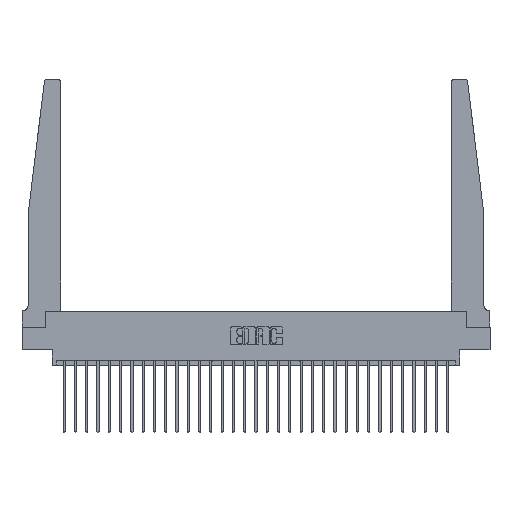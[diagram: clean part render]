
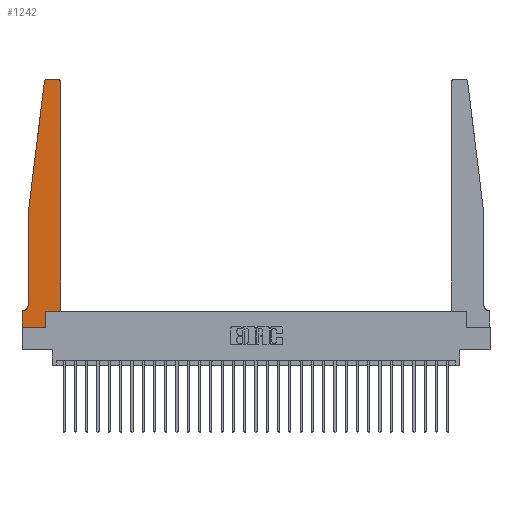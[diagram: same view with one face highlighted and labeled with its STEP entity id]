
A CAD part, top view. The second image highlights one B-rep face of the part: STEP entity #1242.
In plain terms, the highlighted planar face has unit normal (0, 0, 1).
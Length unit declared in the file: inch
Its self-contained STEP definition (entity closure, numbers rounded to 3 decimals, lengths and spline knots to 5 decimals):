
#350 = EDGE_CURVE ( 'NONE', #8178, #1044, #15282, .T. ) ;
#529 = VECTOR ( 'NONE', #13873, 39.37008 ) ;
#693 = LINE ( 'NONE', #27431, #7418 ) ;
#1044 = VERTEX_POINT ( 'NONE', #14270 ) ;
#1242 = ADVANCED_FACE ( 'NONE', ( #22518 ), #8789, .T. ) ;
#1253 = CARTESIAN_POINT ( 'NONE',  ( 0.065, 0.1875, 0.37 ) ) ;
#1385 = CARTESIAN_POINT ( 'NONE',  ( 0.425, 2.72, 0.37 ) ) ;
#1586 = AXIS2_PLACEMENT_3D ( 'NONE', #4360, #19884, #4650 ) ;
#1674 = AXIS2_PLACEMENT_3D ( 'NONE', #8197, #3888, #26198 ) ;
#1875 = CARTESIAN_POINT ( 'NONE',  ( 0.065, 1.25, 0.37 ) ) ;
#2654 = CARTESIAN_POINT ( 'NONE',  ( 0.24675, 2.72367, 0.37 ) ) ;
#2753 = CIRCLE ( 'NONE', #22094, 0.05 ) ;
#3309 = CARTESIAN_POINT ( 'NONE',  ( 0.2605, 0.18, 0.37 ) ) ;
#3790 = DIRECTION ( 'NONE',  ( 1., 0., 0. ) ) ;
#3842 = VECTOR ( 'NONE', #3790, 39.37008 ) ;
#3888 = DIRECTION ( 'NONE',  ( 0., 0., 1. ) ) ;
#4136 = CARTESIAN_POINT ( 'NONE',  ( 0.395, 2.75, 0.37 ) ) ;
#4234 = EDGE_CURVE ( 'NONE', #24091, #22727, #22936, .T. ) ;
#4360 = CARTESIAN_POINT ( 'NONE',  ( 0., 0.1875, 0.37 ) ) ;
#4423 = CARTESIAN_POINT ( 'NONE',  ( 0.065, 1.25, 0.37 ) ) ;
#4650 = DIRECTION ( 'NONE',  ( 1., 0., 0. ) ) ;
#5413 = CARTESIAN_POINT ( 'NONE',  ( 0.27653, 2.75, 0.37 ) ) ;
#5440 = CARTESIAN_POINT ( 'NONE',  ( 0., 0., 0.37 ) ) ;
#6039 = EDGE_CURVE ( 'NONE', #22727, #13927, #14411, .T. ) ;
#6421 = EDGE_CURVE ( 'NONE', #1044, #10842, #12146, .T. ) ;
#6954 = ORIENTED_EDGE ( 'NONE', *, *, #12578, .T. ) ;
#7418 = VECTOR ( 'NONE', #26884, 39.37008 ) ;
#8098 = LINE ( 'NONE', #5440, #3842 ) ;
#8162 = CARTESIAN_POINT ( 'NONE',  ( 0., 0., 0.37 ) ) ;
#8178 = VERTEX_POINT ( 'NONE', #20842 ) ;
#8197 = CARTESIAN_POINT ( 'NONE',  ( 0.395, 2.72, 0.37 ) ) ;
#8360 = LINE ( 'NONE', #26232, #26823 ) ;
#8573 = CIRCLE ( 'NONE', #25087, 0.03 ) ;
#8661 = ORIENTED_EDGE ( 'NONE', *, *, #4234, .T. ) ;
#8789 = PLANE ( 'NONE',  #1586 ) ;
#8797 = DIRECTION ( 'NONE',  ( 1., 0., 0. ) ) ;
#9019 = VERTEX_POINT ( 'NONE', #4423 ) ;
#9257 = LINE ( 'NONE', #1875, #20826 ) ;
#9444 = VECTOR ( 'NONE', #24991, 39.37008 ) ;
#9929 = EDGE_LOOP ( 'NONE', ( #18890, #26732, #19104, #17095, #13205, #13146, #19333, #11712, #20297, #6954, #8661, #21748 ) ) ;
#10842 = VERTEX_POINT ( 'NONE', #22408 ) ;
#11411 = CARTESIAN_POINT ( 'NONE',  ( 0.2605, 0.18, 0.37 ) ) ;
#11477 = VERTEX_POINT ( 'NONE', #3309 ) ;
#11512 = LINE ( 'NONE', #27296, #529 ) ;
#11712 = ORIENTED_EDGE ( 'NONE', *, *, #17496, .T. ) ;
#12146 = LINE ( 'NONE', #8162, #19384 ) ;
#12231 = CARTESIAN_POINT ( 'NONE',  ( 0.27653, 2.72, 0.37 ) ) ;
#12578 = EDGE_CURVE ( 'NONE', #11477, #24091, #8360, .T. ) ;
#13099 = DIRECTION ( 'NONE',  ( -1., 0., 0. ) ) ;
#13146 = ORIENTED_EDGE ( 'NONE', *, *, #350, .T. ) ;
#13205 = ORIENTED_EDGE ( 'NONE', *, *, #25623, .T. ) ;
#13873 = DIRECTION ( 'NONE',  ( 0., -1., 0. ) ) ;
#13927 = VERTEX_POINT ( 'NONE', #4136 ) ;
#14072 = CARTESIAN_POINT ( 'NONE',  ( 0.425, 0.18, 0.37 ) ) ;
#14135 = VERTEX_POINT ( 'NONE', #5413 ) ;
#14270 = CARTESIAN_POINT ( 'NONE',  ( 0., 0.1875, 0.37 ) ) ;
#14411 = CIRCLE ( 'NONE', #1674, 0.03 ) ;
#14891 = CARTESIAN_POINT ( 'NONE',  ( 0.2605, 0., 0.37 ) ) ;
#15282 = LINE ( 'NONE', #1253, #24524 ) ;
#15860 = CARTESIAN_POINT ( 'NONE',  ( 0.425, 0.18, 0.37 ) ) ;
#17095 = ORIENTED_EDGE ( 'NONE', *, *, #17418, .T. ) ;
#17418 = EDGE_CURVE ( 'NONE', #9019, #17997, #11512, .T. ) ;
#17496 = EDGE_CURVE ( 'NONE', #10842, #20495, #8098, .T. ) ;
#17566 = EDGE_CURVE ( 'NONE', #14135, #20289, #8573, .T. ) ;
#17997 = VERTEX_POINT ( 'NONE', #23864 ) ;
#18890 = ORIENTED_EDGE ( 'NONE', *, *, #21978, .T. ) ;
#19104 = ORIENTED_EDGE ( 'NONE', *, *, #29017, .T. ) ;
#19333 = ORIENTED_EDGE ( 'NONE', *, *, #6421, .T. ) ;
#19384 = VECTOR ( 'NONE', #23361, 39.37008 ) ;
#19615 = CARTESIAN_POINT ( 'NONE',  ( 0.015, 0.2375, 0.37 ) ) ;
#19884 = DIRECTION ( 'NONE',  ( 0., 0., 1. ) ) ;
#19916 = DIRECTION ( 'NONE',  ( -0.122, -0.992, 0. ) ) ;
#20289 = VERTEX_POINT ( 'NONE', #2654 ) ;
#20297 = ORIENTED_EDGE ( 'NONE', *, *, #26709, .T. ) ;
#20495 = VERTEX_POINT ( 'NONE', #14891 ) ;
#20826 = VECTOR ( 'NONE', #19916, 39.37008 ) ;
#20842 = CARTESIAN_POINT ( 'NONE',  ( 0.015, 0.1875, 0.37 ) ) ;
#21748 = ORIENTED_EDGE ( 'NONE', *, *, #6039, .T. ) ;
#21978 = EDGE_CURVE ( 'NONE', #13927, #14135, #693, .T. ) ;
#22094 = AXIS2_PLACEMENT_3D ( 'NONE', #19615, #28586, #13099 ) ;
#22408 = CARTESIAN_POINT ( 'NONE',  ( 0., 0., 0.37 ) ) ;
#22518 = FACE_OUTER_BOUND ( 'NONE', #9929, .T. ) ;
#22727 = VERTEX_POINT ( 'NONE', #1385 ) ;
#22936 = LINE ( 'NONE', #14072, #23020 ) ;
#23020 = VECTOR ( 'NONE', #23523, 39.37008 ) ;
#23361 = DIRECTION ( 'NONE',  ( 0., -1., 0. ) ) ;
#23523 = DIRECTION ( 'NONE',  ( 0., 1., 0. ) ) ;
#23864 = CARTESIAN_POINT ( 'NONE',  ( 0.065, 0.2375, 0.37 ) ) ;
#24091 = VERTEX_POINT ( 'NONE', #15860 ) ;
#24303 = DIRECTION ( 'NONE',  ( -1., 0., 0. ) ) ;
#24524 = VECTOR ( 'NONE', #24303, 39.37008 ) ;
#24703 = LINE ( 'NONE', #11411, #9444 ) ;
#24991 = DIRECTION ( 'NONE',  ( 0., 1., 0. ) ) ;
#25087 = AXIS2_PLACEMENT_3D ( 'NONE', #12231, #28012, #25811 ) ;
#25623 = EDGE_CURVE ( 'NONE', #17997, #8178, #2753, .T. ) ;
#25811 = DIRECTION ( 'NONE',  ( 1., 0., 0. ) ) ;
#26198 = DIRECTION ( 'NONE',  ( 1., 0., 0. ) ) ;
#26232 = CARTESIAN_POINT ( 'NONE',  ( 0.425, 0.18, 0.37 ) ) ;
#26709 = EDGE_CURVE ( 'NONE', #20495, #11477, #24703, .T. ) ;
#26732 = ORIENTED_EDGE ( 'NONE', *, *, #17566, .T. ) ;
#26823 = VECTOR ( 'NONE', #8797, 39.37008 ) ;
#26884 = DIRECTION ( 'NONE',  ( -1., 0., 0. ) ) ;
#27296 = CARTESIAN_POINT ( 'NONE',  ( 0.065, 1.25, 0.37 ) ) ;
#27431 = CARTESIAN_POINT ( 'NONE',  ( 0.25, 2.75, 0.37 ) ) ;
#28012 = DIRECTION ( 'NONE',  ( 0., 0., 1. ) ) ;
#28586 = DIRECTION ( 'NONE',  ( 0., 0., -1. ) ) ;
#29017 = EDGE_CURVE ( 'NONE', #20289, #9019, #9257, .T. ) ;
